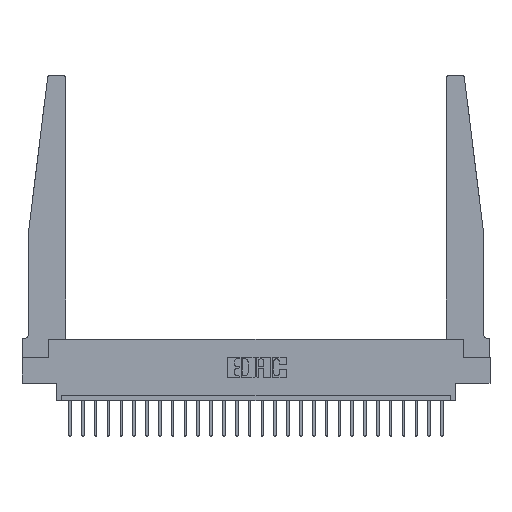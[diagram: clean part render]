
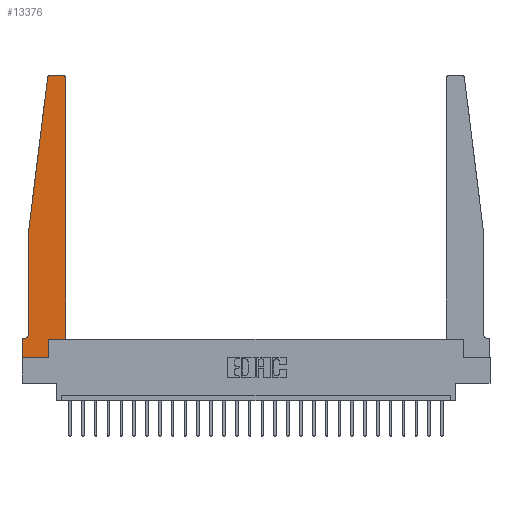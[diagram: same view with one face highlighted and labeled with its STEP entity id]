
A CAD part, top view. The second image highlights one B-rep face of the part: STEP entity #13376.
In plain terms, the highlighted planar face has unit normal (0, 0, 1).
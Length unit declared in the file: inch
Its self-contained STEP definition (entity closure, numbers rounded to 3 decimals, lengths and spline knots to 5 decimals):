
#185 = VERTEX_POINT ( 'NONE', #19086 ) ;
#576 = ORIENTED_EDGE ( 'NONE', *, *, #18111, .T. ) ;
#711 = CARTESIAN_POINT ( 'NONE',  ( 0.2605, 0.18, 0.37 ) ) ;
#951 = ORIENTED_EDGE ( 'NONE', *, *, #11131, .T. ) ;
#959 = CARTESIAN_POINT ( 'NONE',  ( 0.395, 2.75, 0.37 ) ) ;
#1119 = VECTOR ( 'NONE', #12804, 39.37008 ) ;
#1135 = VERTEX_POINT ( 'NONE', #16214 ) ;
#1170 = PLANE ( 'NONE',  #10754 ) ;
#1259 = EDGE_CURVE ( 'NONE', #15805, #1135, #22130, .T. ) ;
#1724 = CARTESIAN_POINT ( 'NONE',  ( 0.395, 2.72, 0.37 ) ) ;
#1804 = CIRCLE ( 'NONE', #19187, 0.03 ) ;
#1892 = VECTOR ( 'NONE', #16178, 39.37008 ) ;
#1943 = CARTESIAN_POINT ( 'NONE',  ( 0.015, 0.1875, 0.37 ) ) ;
#2527 = EDGE_CURVE ( 'NONE', #12142, #18913, #3838, .T. ) ;
#2613 = VERTEX_POINT ( 'NONE', #24104 ) ;
#2780 = DIRECTION ( 'NONE',  ( 1., 0., 0. ) ) ;
#3016 = CARTESIAN_POINT ( 'NONE',  ( 0., 0., 0.37 ) ) ;
#3045 = CARTESIAN_POINT ( 'NONE',  ( 0.425, 0.18, 0.37 ) ) ;
#3109 = DIRECTION ( 'NONE',  ( 1., 0., 0. ) ) ;
#3402 = EDGE_LOOP ( 'NONE', ( #18289, #16378, #10675, #6132, #18729, #18907, #7563, #9802, #576, #18761, #951, #19490 ) ) ;
#3613 = VECTOR ( 'NONE', #16876, 39.37008 ) ;
#3838 = CIRCLE ( 'NONE', #24196, 0.03 ) ;
#4517 = LINE ( 'NONE', #22853, #3613 ) ;
#4572 = EDGE_CURVE ( 'NONE', #9911, #25012, #15347, .T. ) ;
#5086 = DIRECTION ( 'NONE',  ( 1., 0., 0. ) ) ;
#5196 = CIRCLE ( 'NONE', #23462, 0.05 ) ;
#6132 = ORIENTED_EDGE ( 'NONE', *, *, #14299, .T. ) ;
#6192 = DIRECTION ( 'NONE',  ( 0., 1., 0. ) ) ;
#6787 = DIRECTION ( 'NONE',  ( -1., 0., 0. ) ) ;
#7214 = VERTEX_POINT ( 'NONE', #1943 ) ;
#7536 = LINE ( 'NONE', #17849, #12116 ) ;
#7563 = ORIENTED_EDGE ( 'NONE', *, *, #4572, .T. ) ;
#9099 = CARTESIAN_POINT ( 'NONE',  ( 0.065, 1.25, 0.37 ) ) ;
#9105 = LINE ( 'NONE', #23625, #17652 ) ;
#9742 = EDGE_CURVE ( 'NONE', #7214, #9911, #9105, .T. ) ;
#9778 = DIRECTION ( 'NONE',  ( 0., 0., 1. ) ) ;
#9802 = ORIENTED_EDGE ( 'NONE', *, *, #13885, .T. ) ;
#9911 = VERTEX_POINT ( 'NONE', #24227 ) ;
#10034 = DIRECTION ( 'NONE',  ( -1., 0., 0. ) ) ;
#10331 = CARTESIAN_POINT ( 'NONE',  ( 0.25, 2.75, 0.37 ) ) ;
#10461 = DIRECTION ( 'NONE',  ( 0., 0., -1. ) ) ;
#10675 = ORIENTED_EDGE ( 'NONE', *, *, #23162, .T. ) ;
#10754 = AXIS2_PLACEMENT_3D ( 'NONE', #14803, #16756, #5086 ) ;
#11131 = EDGE_CURVE ( 'NONE', #1135, #17401, #4517, .T. ) ;
#11258 = DIRECTION ( 'NONE',  ( 0., -1., 0. ) ) ;
#12116 = VECTOR ( 'NONE', #6192, 39.37008 ) ;
#12142 = VERTEX_POINT ( 'NONE', #12571 ) ;
#12284 = DIRECTION ( 'NONE',  ( 0., 0., 1. ) ) ;
#12449 = EDGE_CURVE ( 'NONE', #17401, #21153, #1804, .T. ) ;
#12571 = CARTESIAN_POINT ( 'NONE',  ( 0.27653, 2.75, 0.37 ) ) ;
#12804 = DIRECTION ( 'NONE',  ( -0.122, -0.992, 0. ) ) ;
#12838 = CARTESIAN_POINT ( 'NONE',  ( 0.425, 2.72, 0.37 ) ) ;
#13376 = ADVANCED_FACE ( 'NONE', ( #22616 ), #1170, .T. ) ;
#13778 = DIRECTION ( 'NONE',  ( 1., 0., 0. ) ) ;
#13885 = EDGE_CURVE ( 'NONE', #25012, #17845, #17178, .T. ) ;
#14097 = EDGE_CURVE ( 'NONE', #21153, #12142, #17743, .T. ) ;
#14299 = EDGE_CURVE ( 'NONE', #185, #2613, #19522, .T. ) ;
#14437 = CARTESIAN_POINT ( 'NONE',  ( 0., 0., 0.37 ) ) ;
#14803 = CARTESIAN_POINT ( 'NONE',  ( 0., 0.1875, 0.37 ) ) ;
#15347 = LINE ( 'NONE', #14437, #1892 ) ;
#15805 = VERTEX_POINT ( 'NONE', #711 ) ;
#15963 = EDGE_CURVE ( 'NONE', #2613, #7214, #5196, .T. ) ;
#16176 = DIRECTION ( 'NONE',  ( 1., 0., 0. ) ) ;
#16178 = DIRECTION ( 'NONE',  ( 0., -1., 0. ) ) ;
#16214 = CARTESIAN_POINT ( 'NONE',  ( 0.425, 0.18, 0.37 ) ) ;
#16337 = LINE ( 'NONE', #22589, #1119 ) ;
#16378 = ORIENTED_EDGE ( 'NONE', *, *, #2527, .T. ) ;
#16756 = DIRECTION ( 'NONE',  ( 0., 0., 1. ) ) ;
#16876 = DIRECTION ( 'NONE',  ( 0., 1., 0. ) ) ;
#16894 = DIRECTION ( 'NONE',  ( -1., 0., 0. ) ) ;
#17178 = LINE ( 'NONE', #3016, #21688 ) ;
#17401 = VERTEX_POINT ( 'NONE', #12838 ) ;
#17458 = VECTOR ( 'NONE', #6787, 39.37008 ) ;
#17652 = VECTOR ( 'NONE', #10034, 39.37008 ) ;
#17743 = LINE ( 'NONE', #10331, #17458 ) ;
#17845 = VERTEX_POINT ( 'NONE', #21140 ) ;
#17849 = CARTESIAN_POINT ( 'NONE',  ( 0.2605, 0.18, 0.37 ) ) ;
#17902 = VECTOR ( 'NONE', #2780, 39.37008 ) ;
#18111 = EDGE_CURVE ( 'NONE', #17845, #15805, #7536, .T. ) ;
#18289 = ORIENTED_EDGE ( 'NONE', *, *, #14097, .T. ) ;
#18729 = ORIENTED_EDGE ( 'NONE', *, *, #15963, .T. ) ;
#18761 = ORIENTED_EDGE ( 'NONE', *, *, #1259, .T. ) ;
#18907 = ORIENTED_EDGE ( 'NONE', *, *, #9742, .T. ) ;
#18913 = VERTEX_POINT ( 'NONE', #22606 ) ;
#19086 = CARTESIAN_POINT ( 'NONE',  ( 0.065, 1.25, 0.37 ) ) ;
#19187 = AXIS2_PLACEMENT_3D ( 'NONE', #1724, #9778, #13778 ) ;
#19490 = ORIENTED_EDGE ( 'NONE', *, *, #12449, .T. ) ;
#19522 = LINE ( 'NONE', #9099, #21061 ) ;
#21061 = VECTOR ( 'NONE', #11258, 39.37008 ) ;
#21140 = CARTESIAN_POINT ( 'NONE',  ( 0.2605, 0., 0.37 ) ) ;
#21153 = VERTEX_POINT ( 'NONE', #959 ) ;
#21293 = CARTESIAN_POINT ( 'NONE',  ( 0., 0., 0.37 ) ) ;
#21688 = VECTOR ( 'NONE', #3109, 39.37008 ) ;
#22116 = CARTESIAN_POINT ( 'NONE',  ( 0.015, 0.2375, 0.37 ) ) ;
#22130 = LINE ( 'NONE', #3045, #17902 ) ;
#22589 = CARTESIAN_POINT ( 'NONE',  ( 0.065, 1.25, 0.37 ) ) ;
#22606 = CARTESIAN_POINT ( 'NONE',  ( 0.24675, 2.72367, 0.37 ) ) ;
#22616 = FACE_OUTER_BOUND ( 'NONE', #3402, .T. ) ;
#22853 = CARTESIAN_POINT ( 'NONE',  ( 0.425, 0.18, 0.37 ) ) ;
#23162 = EDGE_CURVE ( 'NONE', #18913, #185, #16337, .T. ) ;
#23462 = AXIS2_PLACEMENT_3D ( 'NONE', #22116, #10461, #16894 ) ;
#23625 = CARTESIAN_POINT ( 'NONE',  ( 0.065, 0.1875, 0.37 ) ) ;
#24104 = CARTESIAN_POINT ( 'NONE',  ( 0.065, 0.2375, 0.37 ) ) ;
#24129 = CARTESIAN_POINT ( 'NONE',  ( 0.27653, 2.72, 0.37 ) ) ;
#24196 = AXIS2_PLACEMENT_3D ( 'NONE', #24129, #12284, #16176 ) ;
#24227 = CARTESIAN_POINT ( 'NONE',  ( 0., 0.1875, 0.37 ) ) ;
#25012 = VERTEX_POINT ( 'NONE', #21293 ) ;
